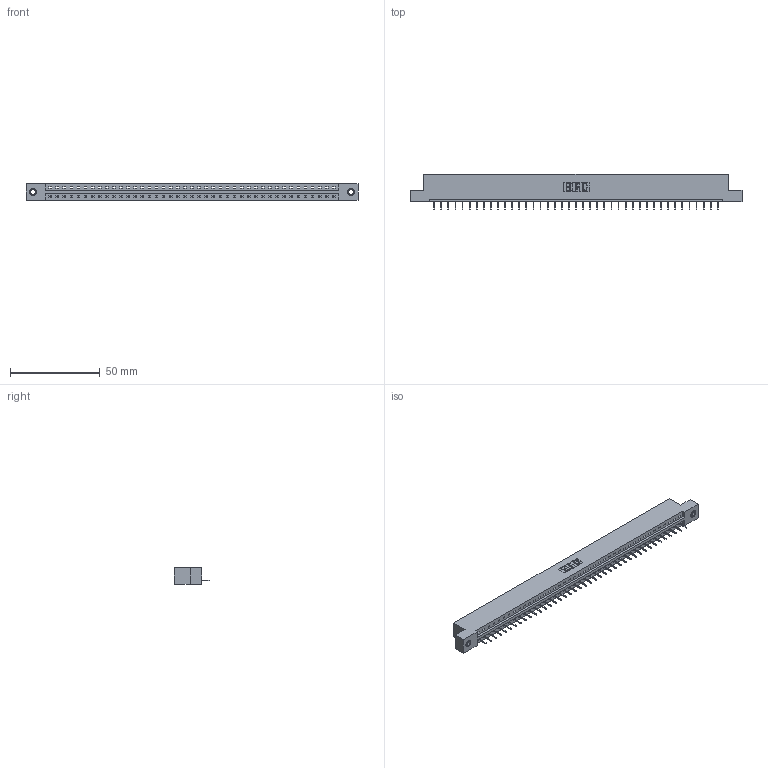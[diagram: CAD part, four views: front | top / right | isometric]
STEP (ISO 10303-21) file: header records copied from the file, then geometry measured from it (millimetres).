
FILE_DESCRIPTION (( 'STEP AP203' ), '1' );
FILE_NAME ('337-041-524-107.STEP', '2018-08-08T21:39:44', ( '' ), ( '' ), 'SwSTEP 2.0', 'SolidWorks 2016', '' );
FILE_SCHEMA (( 'CONFIG_CONTROL_DESIGN' ));
Length unit declared in the file: inch
Products named in the file (4): 337 Part_Flush Mounting Lugs - 0.156 Dia-TI; 345-292-001_345-293-124; 345-250-001_345-250-005-103; 337-041-524-107
Assembly tree (44 placements, depth 2):
  337-041-524-107
    337 Part_Flush Mounting Lugs - 0.156 Dia-TI
    345-292-001_345-293-124  x41
    345-250-001_345-250-005-103  x2
Bounding box: 185.47 x 19.69 x 9.4 mm (x, y, z)
Volume: 19088.6 mm3; surface area: 19191.2 mm2
Topology: 44 solids, 44 shells, 2880 faces, 8319 edges, 5374 vertices
Faces by surface type: plane 2234, cylinder 630, cone 12, torus 4
Entity records: 31866 total; most frequent: CARTESIAN_POINT 5528, ORIENTED_EDGE 5498, DIRECTION 4689, EDGE_CURVE 2749, LINE 2605, VECTOR 2605, VERTEX_POINT 1824, AXIS2_PLACEMENT_3D 1042
